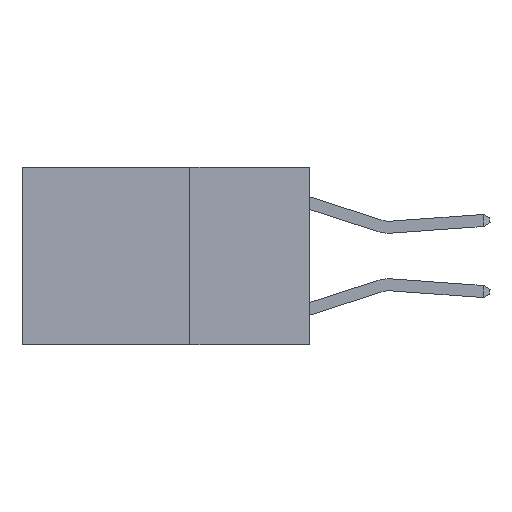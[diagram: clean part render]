
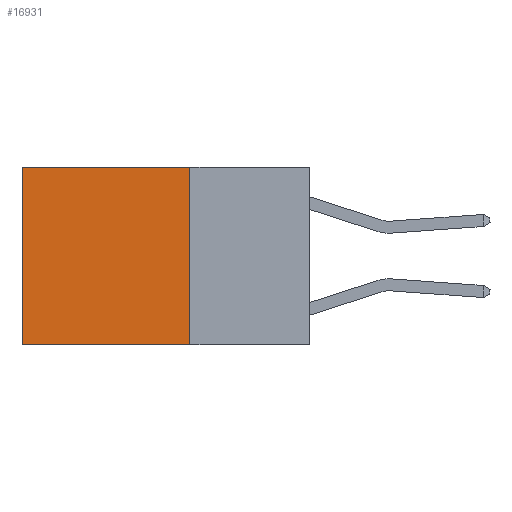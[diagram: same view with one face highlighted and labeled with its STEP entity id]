
A CAD part, left-side view. The second image highlights one B-rep face of the part: STEP entity #16931.
In plain terms, the highlighted planar face has unit normal (-1, 0, 0).
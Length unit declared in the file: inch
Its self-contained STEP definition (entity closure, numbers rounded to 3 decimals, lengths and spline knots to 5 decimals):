
#668 = DIRECTION ( 'NONE',  ( 0., 0., -1. ) ) ;
#1751 = EDGE_CURVE ( 'NONE', #20271, #20475, #7721, .T. ) ;
#2428 = ORIENTED_EDGE ( 'NONE', *, *, #15321, .F. ) ;
#2561 = PLANE ( 'NONE',  #6849 ) ;
#4834 = ORIENTED_EDGE ( 'NONE', *, *, #1751, .T. ) ;
#4966 = VERTEX_POINT ( 'NONE', #17801 ) ;
#6849 = AXIS2_PLACEMENT_3D ( 'NONE', #22815, #9982, #668 ) ;
#7057 = EDGE_LOOP ( 'NONE', ( #4834, #2428, #8347, #19056 ) ) ;
#7721 = LINE ( 'NONE', #22201, #15649 ) ;
#8347 = ORIENTED_EDGE ( 'NONE', *, *, #17028, .F. ) ;
#8561 = CARTESIAN_POINT ( 'NONE',  ( 0.2625, 0.25, 0. ) ) ;
#8797 = CARTESIAN_POINT ( 'NONE',  ( 0.2625, 0.6, 0. ) ) ;
#9218 = DIRECTION ( 'NONE',  ( 0., 1., 0. ) ) ;
#9982 = DIRECTION ( 'NONE',  ( 1., 0., 0. ) ) ;
#10450 = LINE ( 'NONE', #8561, #20521 ) ;
#10932 = LINE ( 'NONE', #18158, #18151 ) ;
#11199 = VERTEX_POINT ( 'NONE', #19329 ) ;
#12846 = DIRECTION ( 'NONE',  ( 0., 1., 0. ) ) ;
#15321 = EDGE_CURVE ( 'NONE', #4966, #20475, #10932, .T. ) ;
#15596 = FACE_OUTER_BOUND ( 'NONE', #7057, .T. ) ;
#15649 = VECTOR ( 'NONE', #21846, 39.37008 ) ;
#16494 = VECTOR ( 'NONE', #9218, 39.37008 ) ;
#16931 = ADVANCED_FACE ( 'NONE', ( #15596 ), #2561, .F. ) ;
#17012 = CARTESIAN_POINT ( 'NONE',  ( 0.2625, 0.6, -0.37 ) ) ;
#17028 = EDGE_CURVE ( 'NONE', #11199, #4966, #10450, .T. ) ;
#17801 = CARTESIAN_POINT ( 'NONE',  ( 0.2625, 0.25, -0.37 ) ) ;
#18151 = VECTOR ( 'NONE', #12846, 39.37008 ) ;
#18158 = CARTESIAN_POINT ( 'NONE',  ( 0.2625, 0.25, -0.37 ) ) ;
#18235 = CARTESIAN_POINT ( 'NONE',  ( 0.2625, 0.25, 0. ) ) ;
#19056 = ORIENTED_EDGE ( 'NONE', *, *, #22750, .T. ) ;
#19329 = CARTESIAN_POINT ( 'NONE',  ( 0.2625, 0.25, 0. ) ) ;
#20152 = LINE ( 'NONE', #18235, #16494 ) ;
#20271 = VERTEX_POINT ( 'NONE', #8797 ) ;
#20475 = VERTEX_POINT ( 'NONE', #17012 ) ;
#20521 = VECTOR ( 'NONE', #21159, 39.37008 ) ;
#21159 = DIRECTION ( 'NONE',  ( 0., 0., -1. ) ) ;
#21846 = DIRECTION ( 'NONE',  ( 0., 0., -1. ) ) ;
#22201 = CARTESIAN_POINT ( 'NONE',  ( 0.2625, 0.6, 0. ) ) ;
#22750 = EDGE_CURVE ( 'NONE', #11199, #20271, #20152, .T. ) ;
#22815 = CARTESIAN_POINT ( 'NONE',  ( 0.2625, 0.25, 0. ) ) ;
